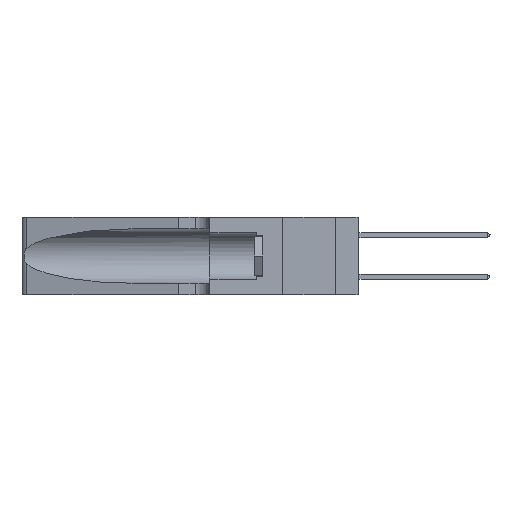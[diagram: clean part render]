
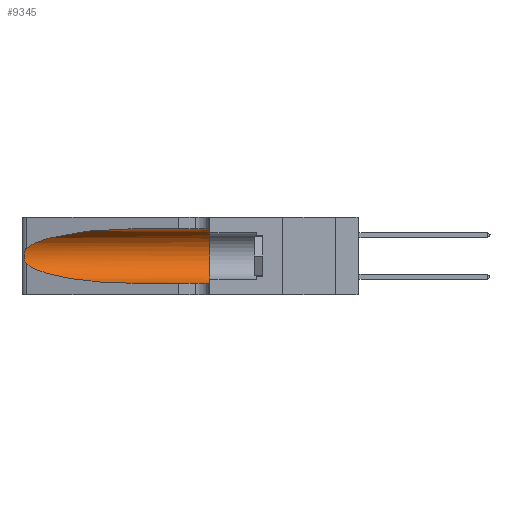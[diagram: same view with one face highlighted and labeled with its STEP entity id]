
A CAD part, left-side view. The second image highlights one B-rep face of the part: STEP entity #9345.
In plain terms, the highlighted cylindrical face has radius 3.308 mm (diameter 6.617 mm), a partial arc.
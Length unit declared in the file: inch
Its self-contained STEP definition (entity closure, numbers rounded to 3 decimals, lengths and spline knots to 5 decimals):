
#94 = DIRECTION ( 'NONE',  ( 0., 0., -1. ) ) ;
#282 = CARTESIAN_POINT ( 'NONE',  ( 0.25555, 1.22994, 0.2215 ) ) ;
#370 = CARTESIAN_POINT ( 'NONE',  ( 0.25487, 1.22718, 0.14631 ) ) ;
#405 = CARTESIAN_POINT ( 'NONE',  ( 0.1305, 0.72297, 0.05475 ) ) ;
#1463 = CARTESIAN_POINT ( 'NONE',  ( 0.1305, 0.72297, 0.05475 ) ) ;
#1880 = LINE ( 'NONE', #24374, #16719 ) ;
#2118 = ORIENTED_EDGE ( 'NONE', *, *, #5378, .T. ) ;
#2275 = CARTESIAN_POINT ( 'NONE',  ( 0.25639, 1.23184, 0.21858 ) ) ;
#2569 =( BOUNDED_CURVE ( )  B_SPLINE_CURVE ( 3, ( #24318, #24395, #14993, #3412 ),
 .UNSPECIFIED., .F., .F. ) 
 B_SPLINE_CURVE_WITH_KNOTS ( ( 4, 4 ),
 ( 1.5708, 2.84003 ),
 .UNSPECIFIED. ) 
 CURVE ( )  GEOMETRIC_REPRESENTATION_ITEM ( )  RATIONAL_B_SPLINE_CURVE ( ( 1., 0.87, 0.87, 1. ) ) 
 REPRESENTATION_ITEM ( '' )  );
#3050 =( BOUNDED_CURVE ( )  B_SPLINE_CURVE ( 3, ( #4304, #10166, #12149, #405 ),
 .UNSPECIFIED., .F., .F. ) 
 B_SPLINE_CURVE_WITH_KNOTS ( ( 4, 4 ),
 ( 3.44316, 4.71239 ),
 .UNSPECIFIED. ) 
 CURVE ( )  GEOMETRIC_REPRESENTATION_ITEM ( )  RATIONAL_B_SPLINE_CURVE ( ( 1., 0.87, 0.87, 1. ) ) 
 REPRESENTATION_ITEM ( '' )  );
#3226 = B_SPLINE_CURVE_WITH_KNOTS ( 'NONE', 3,
 ( #13931, #282, #2275, #15835, #4265, #17714, #6223, #19613, #8154, #21508, #10124, #23407, #12105, #370 ),
 .UNSPECIFIED., .F., .F.,
 ( 4, 2, 2, 2, 2, 2, 4 ),
 ( 0., 0.00027, 0.00053, 0.00107, 0.0016, 0.00187, 0.00214 ),
 .UNSPECIFIED. ) ;
#3412 = CARTESIAN_POINT ( 'NONE',  ( 0.25487, 1.22718, 0.22369 ) ) ;
#3790 = LINE ( 'NONE', #13515, #8313 ) ;
#4265 = CARTESIAN_POINT ( 'NONE',  ( 0.25854, 1.2359, 0.20912 ) ) ;
#4304 = CARTESIAN_POINT ( 'NONE',  ( 0.25487, 1.22718, 0.14631 ) ) ;
#5378 = EDGE_CURVE ( 'NONE', #16994, #13704, #3226, .T. ) ;
#6223 = CARTESIAN_POINT ( 'NONE',  ( 0.26075, 1.23896, 0.19203 ) ) ;
#6619 = ORIENTED_EDGE ( 'NONE', *, *, #21629, .F. ) ;
#6684 = EDGE_CURVE ( 'NONE', #13704, #11747, #3050, .T. ) ;
#6829 = FACE_OUTER_BOUND ( 'NONE', #17870, .T. ) ;
#6875 = DIRECTION ( 'NONE',  ( 0., 1., 0. ) ) ;
#7280 = EDGE_CURVE ( 'NONE', #21785, #16994, #2569, .T. ) ;
#7454 = CARTESIAN_POINT ( 'NONE',  ( 0.25487, 1.22718, 0.22369 ) ) ;
#8154 = CARTESIAN_POINT ( 'NONE',  ( 0.26017, 1.23833, 0.17102 ) ) ;
#8313 = VECTOR ( 'NONE', #15422, 39.37008 ) ;
#9134 = AXIS2_PLACEMENT_3D ( 'NONE', #18343, #6875, #20239 ) ;
#9314 = DIRECTION ( 'NONE',  ( 0., -1., 0. ) ) ;
#9345 = ADVANCED_FACE ( 'NONE', ( #6829 ), #21470, .F. ) ;
#9357 = ORIENTED_EDGE ( 'NONE', *, *, #18670, .F. ) ;
#9559 = VERTEX_POINT ( 'NONE', #12348 ) ;
#10124 = CARTESIAN_POINT ( 'NONE',  ( 0.25789, 1.23486, 0.15765 ) ) ;
#10166 = CARTESIAN_POINT ( 'NONE',  ( 0.2373, 1.15595, 0.08982 ) ) ;
#11747 = VERTEX_POINT ( 'NONE', #1463 ) ;
#11851 = CARTESIAN_POINT ( 'NONE',  ( 0.1305, 1.61858, 0.185 ) ) ;
#12105 = CARTESIAN_POINT ( 'NONE',  ( 0.25555, 1.22993, 0.14849 ) ) ;
#12149 = CARTESIAN_POINT ( 'NONE',  ( 0.18966, 0.96281, 0.05475 ) ) ;
#12348 = CARTESIAN_POINT ( 'NONE',  ( 0.1305, 0.35, 0.05475 ) ) ;
#13153 = ORIENTED_EDGE ( 'NONE', *, *, #21124, .T. ) ;
#13515 = CARTESIAN_POINT ( 'NONE',  ( 0.1305, 1.61858, 0.05475 ) ) ;
#13704 = VERTEX_POINT ( 'NONE', #16555 ) ;
#13931 = CARTESIAN_POINT ( 'NONE',  ( 0.25487, 1.22718, 0.22369 ) ) ;
#14993 = CARTESIAN_POINT ( 'NONE',  ( 0.2373, 1.15595, 0.28018 ) ) ;
#15422 = DIRECTION ( 'NONE',  ( 0., -1., 0. ) ) ;
#15829 = CARTESIAN_POINT ( 'NONE',  ( 0.1305, 0.35, 0.31525 ) ) ;
#15835 = CARTESIAN_POINT ( 'NONE',  ( 0.25787, 1.23484, 0.2124 ) ) ;
#16555 = CARTESIAN_POINT ( 'NONE',  ( 0.25487, 1.22718, 0.14631 ) ) ;
#16719 = VECTOR ( 'NONE', #9314, 39.37008 ) ;
#16994 = VERTEX_POINT ( 'NONE', #7454 ) ;
#17467 = DIRECTION ( 'NONE',  ( 0., -1., 0. ) ) ;
#17714 = CARTESIAN_POINT ( 'NONE',  ( 0.26018, 1.23835, 0.19895 ) ) ;
#17786 = AXIS2_PLACEMENT_3D ( 'NONE', #11851, #17467, #94 ) ;
#17870 = EDGE_LOOP ( 'NONE', ( #20143, #2118, #19270, #13153, #9357, #6619 ) ) ;
#18343 = CARTESIAN_POINT ( 'NONE',  ( 0.1305, 0.35, 0.185 ) ) ;
#18670 = EDGE_CURVE ( 'NONE', #19389, #9559, #24796, .T. ) ;
#19270 = ORIENTED_EDGE ( 'NONE', *, *, #6684, .T. ) ;
#19389 = VERTEX_POINT ( 'NONE', #15829 ) ;
#19613 = CARTESIAN_POINT ( 'NONE',  ( 0.26075, 1.23896, 0.178 ) ) ;
#20143 = ORIENTED_EDGE ( 'NONE', *, *, #7280, .T. ) ;
#20239 = DIRECTION ( 'NONE',  ( 0., 0., 1. ) ) ;
#21124 = EDGE_CURVE ( 'NONE', #11747, #9559, #3790, .T. ) ;
#21470 = CYLINDRICAL_SURFACE ( 'NONE', #17786, 0.13025 ) ;
#21508 = CARTESIAN_POINT ( 'NONE',  ( 0.25856, 1.23593, 0.16098 ) ) ;
#21629 = EDGE_CURVE ( 'NONE', #21785, #19389, #1880, .T. ) ;
#21785 = VERTEX_POINT ( 'NONE', #23644 ) ;
#23407 = CARTESIAN_POINT ( 'NONE',  ( 0.25639, 1.23186, 0.15144 ) ) ;
#23644 = CARTESIAN_POINT ( 'NONE',  ( 0.1305, 0.72297, 0.31525 ) ) ;
#24318 = CARTESIAN_POINT ( 'NONE',  ( 0.1305, 0.72297, 0.31525 ) ) ;
#24374 = CARTESIAN_POINT ( 'NONE',  ( 0.1305, 1.61858, 0.31525 ) ) ;
#24395 = CARTESIAN_POINT ( 'NONE',  ( 0.18966, 0.96281, 0.31525 ) ) ;
#24796 = CIRCLE ( 'NONE', #9134, 0.13025 ) ;
